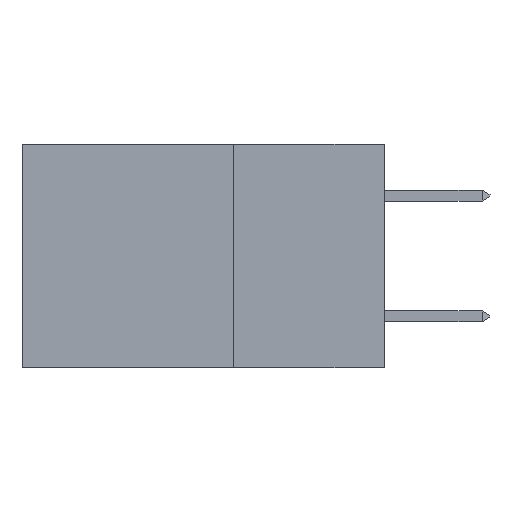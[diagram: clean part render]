
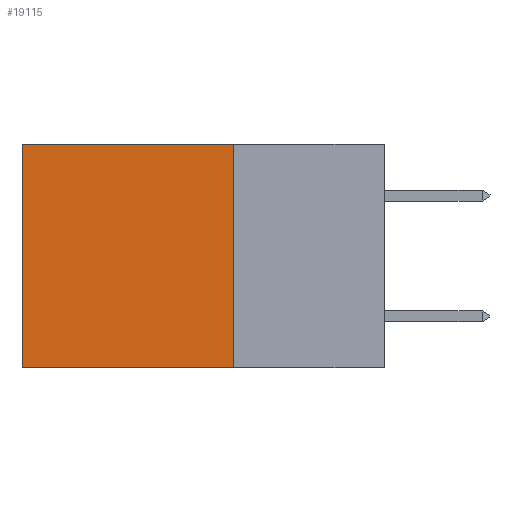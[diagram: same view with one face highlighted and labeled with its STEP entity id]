
A CAD part, left-side view. The second image highlights one B-rep face of the part: STEP entity #19115.
In plain terms, the highlighted planar face has unit normal (-1, 0, 0).
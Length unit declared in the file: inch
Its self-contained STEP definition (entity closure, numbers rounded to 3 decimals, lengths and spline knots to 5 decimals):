
#124 = PLANE ( 'NONE',  #19594 ) ;
#195 = CARTESIAN_POINT ( 'NONE',  ( 0.2875, 0.25, 0. ) ) ;
#948 = VERTEX_POINT ( 'NONE', #16883 ) ;
#1313 = EDGE_CURVE ( 'NONE', #7636, #11927, #14687, .T. ) ;
#1348 = VECTOR ( 'NONE', #7856, 39.37008 ) ;
#2726 = ORIENTED_EDGE ( 'NONE', *, *, #14623, .F. ) ;
#4989 = VECTOR ( 'NONE', #18656, 39.37008 ) ;
#6242 = ORIENTED_EDGE ( 'NONE', *, *, #18372, .T. ) ;
#6437 = EDGE_LOOP ( 'NONE', ( #11551, #15643, #2726, #6242 ) ) ;
#7362 = VECTOR ( 'NONE', #17850, 39.37008 ) ;
#7636 = VERTEX_POINT ( 'NONE', #19232 ) ;
#7856 = DIRECTION ( 'NONE',  ( 0., 0., -1. ) ) ;
#9415 = DIRECTION ( 'NONE',  ( 1., 0., 0. ) ) ;
#10713 = LINE ( 'NONE', #17994, #7362 ) ;
#11551 = ORIENTED_EDGE ( 'NONE', *, *, #14285, .T. ) ;
#11888 = CARTESIAN_POINT ( 'NONE',  ( 0.2875, 0.6, -0.37 ) ) ;
#11927 = VERTEX_POINT ( 'NONE', #11888 ) ;
#13277 = VECTOR ( 'NONE', #14098, 39.37008 ) ;
#14098 = DIRECTION ( 'NONE',  ( 0., 1., 0. ) ) ;
#14285 = EDGE_CURVE ( 'NONE', #948, #11927, #15809, .T. ) ;
#14623 = EDGE_CURVE ( 'NONE', #17846, #7636, #10713, .T. ) ;
#14687 = LINE ( 'NONE', #16960, #4989 ) ;
#15363 = CARTESIAN_POINT ( 'NONE',  ( 0.2875, 0.25, 0. ) ) ;
#15452 = FACE_OUTER_BOUND ( 'NONE', #6437, .T. ) ;
#15643 = ORIENTED_EDGE ( 'NONE', *, *, #1313, .F. ) ;
#15809 = LINE ( 'NONE', #17180, #1348 ) ;
#16883 = CARTESIAN_POINT ( 'NONE',  ( 0.2875, 0.6, 0. ) ) ;
#16960 = CARTESIAN_POINT ( 'NONE',  ( 0.2875, 0.25, -0.37 ) ) ;
#17036 = CARTESIAN_POINT ( 'NONE',  ( 0.2875, 0.25, 0. ) ) ;
#17094 = DIRECTION ( 'NONE',  ( 0., 0., -1. ) ) ;
#17180 = CARTESIAN_POINT ( 'NONE',  ( 0.2875, 0.6, 0. ) ) ;
#17846 = VERTEX_POINT ( 'NONE', #15363 ) ;
#17850 = DIRECTION ( 'NONE',  ( 0., 0., -1. ) ) ;
#17994 = CARTESIAN_POINT ( 'NONE',  ( 0.2875, 0.25, 0. ) ) ;
#18372 = EDGE_CURVE ( 'NONE', #17846, #948, #19781, .T. ) ;
#18656 = DIRECTION ( 'NONE',  ( 0., 1., 0. ) ) ;
#19115 = ADVANCED_FACE ( 'NONE', ( #15452 ), #124, .F. ) ;
#19232 = CARTESIAN_POINT ( 'NONE',  ( 0.2875, 0.25, -0.37 ) ) ;
#19594 = AXIS2_PLACEMENT_3D ( 'NONE', #17036, #9415, #17094 ) ;
#19781 = LINE ( 'NONE', #195, #13277 ) ;
